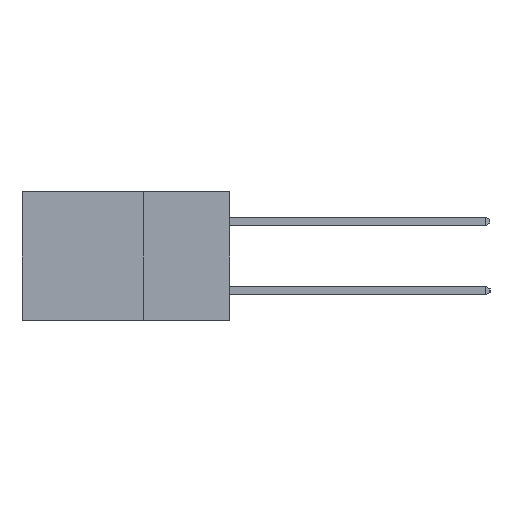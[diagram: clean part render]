
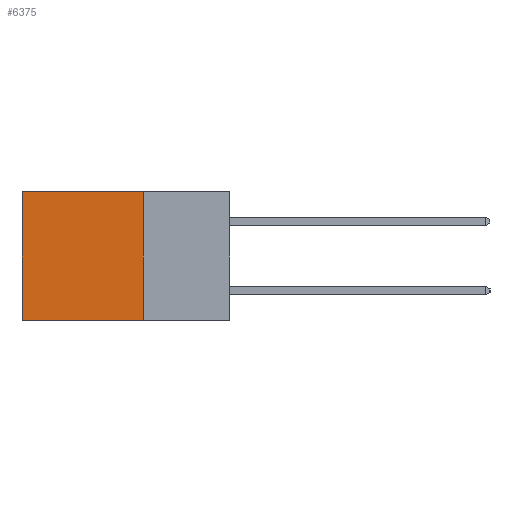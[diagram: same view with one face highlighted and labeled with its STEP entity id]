
A CAD part, left-side view. The second image highlights one B-rep face of the part: STEP entity #6375.
In plain terms, the highlighted planar face has unit normal (-1, 0, 0).
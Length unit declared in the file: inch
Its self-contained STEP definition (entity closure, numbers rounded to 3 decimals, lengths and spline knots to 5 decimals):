
#62 = AXIS2_PLACEMENT_3D ( 'NONE', #3031, #2853, #2851 ) ;
#166 = LINE ( 'NONE', #2663, #4923 ) ;
#181 = VERTEX_POINT ( 'NONE', #9270 ) ;
#241 = DIRECTION ( 'NONE',  ( 0., 0., -1. ) ) ;
#2019 = DIRECTION ( 'NONE',  ( 0., 0., -1. ) ) ;
#2142 = CARTESIAN_POINT ( 'NONE',  ( 0.2615, 0.25, -0.37 ) ) ;
#2516 = DIRECTION ( 'NONE',  ( 0., 1., 0. ) ) ;
#2663 = CARTESIAN_POINT ( 'NONE',  ( 0.2615, 0.25, -0.37 ) ) ;
#2802 = VERTEX_POINT ( 'NONE', #6781 ) ;
#2851 = DIRECTION ( 'NONE',  ( 0., 0., -1. ) ) ;
#2853 = DIRECTION ( 'NONE',  ( 1., 0., 0. ) ) ;
#3031 = CARTESIAN_POINT ( 'NONE',  ( 0.2615, 0.25, -0.37 ) ) ;
#3057 = EDGE_CURVE ( 'NONE', #2802, #4358, #13629, .T. ) ;
#3135 = PLANE ( 'NONE',  #62 ) ;
#3245 = LINE ( 'NONE', #13146, #9117 ) ;
#3425 = DIRECTION ( 'NONE',  ( 0., 1., 0. ) ) ;
#3437 = CARTESIAN_POINT ( 'NONE',  ( 0.2615, 0.25, -0.37 ) ) ;
#4358 = VERTEX_POINT ( 'NONE', #3437 ) ;
#4367 = EDGE_CURVE ( 'NONE', #2802, #6567, #10501, .T. ) ;
#4790 = EDGE_CURVE ( 'NONE', #4358, #181, #166, .T. ) ;
#4923 = VECTOR ( 'NONE', #2516, 39.37008 ) ;
#5260 = ORIENTED_EDGE ( 'NONE', *, *, #12439, .T. ) ;
#5589 = EDGE_LOOP ( 'NONE', ( #5260, #11527, #6114, #13448 ) ) ;
#6114 = ORIENTED_EDGE ( 'NONE', *, *, #3057, .F. ) ;
#6375 = ADVANCED_FACE ( 'NONE', ( #6925 ), #3135, .F. ) ;
#6567 = VERTEX_POINT ( 'NONE', #13041 ) ;
#6781 = CARTESIAN_POINT ( 'NONE',  ( 0.2615, 0.25, 0. ) ) ;
#6925 = FACE_OUTER_BOUND ( 'NONE', #5589, .T. ) ;
#8248 = VECTOR ( 'NONE', #2019, 39.37008 ) ;
#9117 = VECTOR ( 'NONE', #241, 39.37008 ) ;
#9270 = CARTESIAN_POINT ( 'NONE',  ( 0.2615, 0.6, -0.37 ) ) ;
#10295 = CARTESIAN_POINT ( 'NONE',  ( 0.2615, 0.25, 0. ) ) ;
#10501 = LINE ( 'NONE', #10295, #12558 ) ;
#11527 = ORIENTED_EDGE ( 'NONE', *, *, #4790, .F. ) ;
#12439 = EDGE_CURVE ( 'NONE', #6567, #181, #3245, .T. ) ;
#12558 = VECTOR ( 'NONE', #3425, 39.37008 ) ;
#13041 = CARTESIAN_POINT ( 'NONE',  ( 0.2615, 0.6, 0. ) ) ;
#13146 = CARTESIAN_POINT ( 'NONE',  ( 0.2615, 0.6, -0.37 ) ) ;
#13448 = ORIENTED_EDGE ( 'NONE', *, *, #4367, .T. ) ;
#13629 = LINE ( 'NONE', #2142, #8248 ) ;
